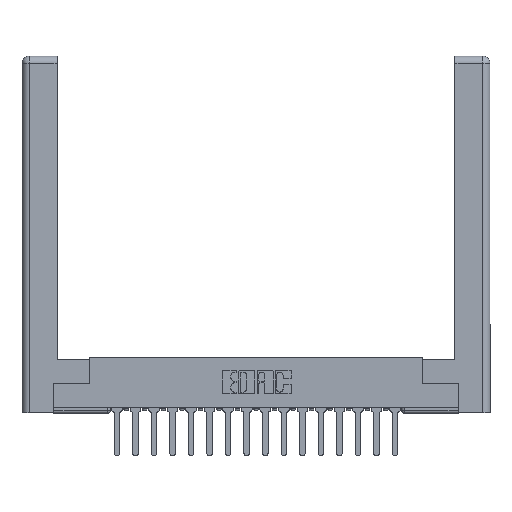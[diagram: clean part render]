
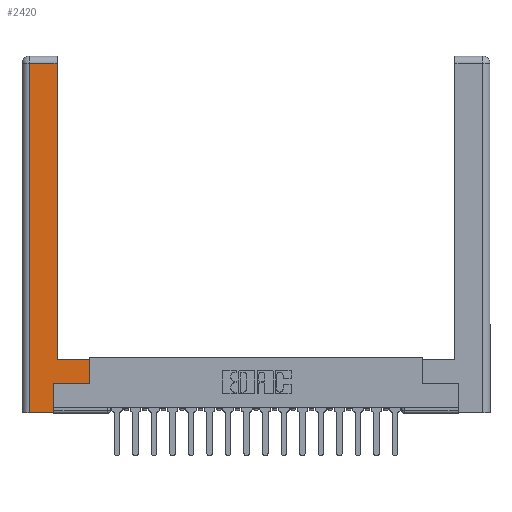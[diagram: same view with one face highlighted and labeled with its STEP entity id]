
A CAD part, top view. The second image highlights one B-rep face of the part: STEP entity #2420.
In plain terms, the highlighted planar face has unit normal (0, 0, 1).
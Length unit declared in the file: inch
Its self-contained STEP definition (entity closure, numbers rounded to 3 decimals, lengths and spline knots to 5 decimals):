
#153 = CARTESIAN_POINT ( 'NONE',  ( 0.265, 0.245, 0. ) ) ;
#638 = DIRECTION ( 'NONE',  ( 0., 1., 0. ) ) ;
#813 = VERTEX_POINT ( 'NONE', #11343 ) ;
#1442 = EDGE_CURVE ( 'NONE', #17904, #13750, #15899, .T. ) ;
#1457 = LINE ( 'NONE', #17834, #18848 ) ;
#1633 = CARTESIAN_POINT ( 'NONE',  ( 0.565, 0.245, 0. ) ) ;
#1903 = VECTOR ( 'NONE', #6594, 39.37008 ) ;
#2182 = VERTEX_POINT ( 'NONE', #13135 ) ;
#2311 = ORIENTED_EDGE ( 'NONE', *, *, #5889, .T. ) ;
#2420 = ADVANCED_FACE ( 'NONE', ( #10061 ), #6966, .F. ) ;
#3121 = LINE ( 'NONE', #6651, #10843 ) ;
#3149 = DIRECTION ( 'NONE',  ( -1., 0., 0. ) ) ;
#3428 = LINE ( 'NONE', #1633, #10683 ) ;
#3564 = AXIS2_PLACEMENT_3D ( 'NONE', #8472, #13478, #3149 ) ;
#3712 = EDGE_CURVE ( 'NONE', #13750, #813, #4687, .T. ) ;
#4269 = EDGE_CURVE ( 'NONE', #18350, #19597, #12951, .T. ) ;
#4384 = EDGE_CURVE ( 'NONE', #813, #18350, #9336, .T. ) ;
#4687 = LINE ( 'NONE', #18846, #5394 ) ;
#4731 = VECTOR ( 'NONE', #4800, 39.37008 ) ;
#4800 = DIRECTION ( 'NONE',  ( 0., -1., 0. ) ) ;
#5394 = VECTOR ( 'NONE', #6462, 39.37008 ) ;
#5889 = EDGE_CURVE ( 'NONE', #2182, #10479, #10008, .T. ) ;
#6381 = ORIENTED_EDGE ( 'NONE', *, *, #4269, .T. ) ;
#6462 = DIRECTION ( 'NONE',  ( 0., 1., 0. ) ) ;
#6594 = DIRECTION ( 'NONE',  ( -1., 0., 0. ) ) ;
#6651 = CARTESIAN_POINT ( 'NONE',  ( 0.565, 0.45, 0. ) ) ;
#6678 = CARTESIAN_POINT ( 'NONE',  ( 0.0615, 2.94, 0. ) ) ;
#6720 = CARTESIAN_POINT ( 'NONE',  ( 0.295, 0.45, 0. ) ) ;
#6966 = PLANE ( 'NONE',  #3564 ) ;
#7629 = DIRECTION ( 'NONE',  ( 1., 0., 0. ) ) ;
#8256 = EDGE_CURVE ( 'NONE', #10479, #18177, #3428, .T. ) ;
#8472 = CARTESIAN_POINT ( 'NONE',  ( 0., 0., 0. ) ) ;
#9336 = LINE ( 'NONE', #6678, #10802 ) ;
#9368 = EDGE_CURVE ( 'NONE', #18177, #17904, #3121, .T. ) ;
#9510 = CARTESIAN_POINT ( 'NONE',  ( 0.265, 0.245, 0. ) ) ;
#9645 = ORIENTED_EDGE ( 'NONE', *, *, #4384, .T. ) ;
#10008 = LINE ( 'NONE', #153, #17522 ) ;
#10061 = FACE_OUTER_BOUND ( 'NONE', #17855, .T. ) ;
#10479 = VERTEX_POINT ( 'NONE', #9510 ) ;
#10522 = CARTESIAN_POINT ( 'NONE',  ( 0.565, 0.45, 0. ) ) ;
#10683 = VECTOR ( 'NONE', #7629, 39.37008 ) ;
#10802 = VECTOR ( 'NONE', #17507, 39.37008 ) ;
#10843 = VECTOR ( 'NONE', #638, 39.37008 ) ;
#11343 = CARTESIAN_POINT ( 'NONE',  ( 0.295, 2.94, 0. ) ) ;
#12544 = ORIENTED_EDGE ( 'NONE', *, *, #1442, .T. ) ;
#12848 = CARTESIAN_POINT ( 'NONE',  ( 0.0615, 0., 0. ) ) ;
#12951 = LINE ( 'NONE', #13995, #4731 ) ;
#13135 = CARTESIAN_POINT ( 'NONE',  ( 0.265, 0., 0. ) ) ;
#13478 = DIRECTION ( 'NONE',  ( 0., 0., -1. ) ) ;
#13750 = VERTEX_POINT ( 'NONE', #19152 ) ;
#13810 = ORIENTED_EDGE ( 'NONE', *, *, #8256, .T. ) ;
#13995 = CARTESIAN_POINT ( 'NONE',  ( 0.0615, 0., 0. ) ) ;
#14806 = DIRECTION ( 'NONE',  ( 1., 0., 0. ) ) ;
#15677 = EDGE_CURVE ( 'NONE', #19597, #2182, #1457, .T. ) ;
#15762 = DIRECTION ( 'NONE',  ( 0., 1., 0. ) ) ;
#15899 = LINE ( 'NONE', #6720, #1903 ) ;
#16219 = CARTESIAN_POINT ( 'NONE',  ( 0.0615, 2.94, 0. ) ) ;
#17507 = DIRECTION ( 'NONE',  ( -1., 0., 0. ) ) ;
#17522 = VECTOR ( 'NONE', #15762, 39.37008 ) ;
#17670 = ORIENTED_EDGE ( 'NONE', *, *, #9368, .T. ) ;
#17736 = ORIENTED_EDGE ( 'NONE', *, *, #15677, .T. ) ;
#17834 = CARTESIAN_POINT ( 'NONE',  ( 0.265, 0., 0. ) ) ;
#17855 = EDGE_LOOP ( 'NONE', ( #18016, #9645, #6381, #17736, #2311, #13810, #17670, #12544 ) ) ;
#17904 = VERTEX_POINT ( 'NONE', #10522 ) ;
#18016 = ORIENTED_EDGE ( 'NONE', *, *, #3712, .T. ) ;
#18177 = VERTEX_POINT ( 'NONE', #19129 ) ;
#18350 = VERTEX_POINT ( 'NONE', #16219 ) ;
#18846 = CARTESIAN_POINT ( 'NONE',  ( 0.295, 3., 0. ) ) ;
#18848 = VECTOR ( 'NONE', #14806, 39.37008 ) ;
#19129 = CARTESIAN_POINT ( 'NONE',  ( 0.565, 0.245, 0. ) ) ;
#19152 = CARTESIAN_POINT ( 'NONE',  ( 0.295, 0.45, 0. ) ) ;
#19597 = VERTEX_POINT ( 'NONE', #12848 ) ;
